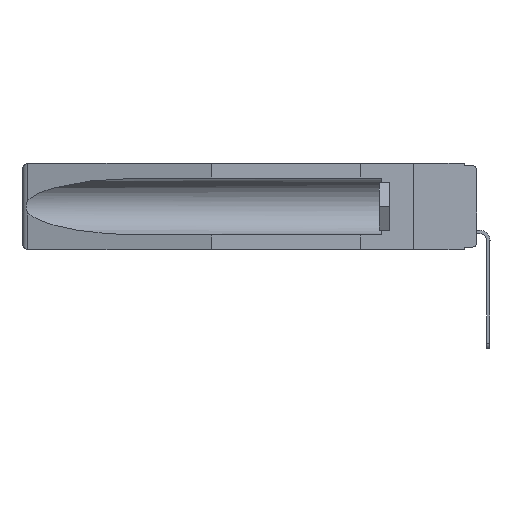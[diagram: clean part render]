
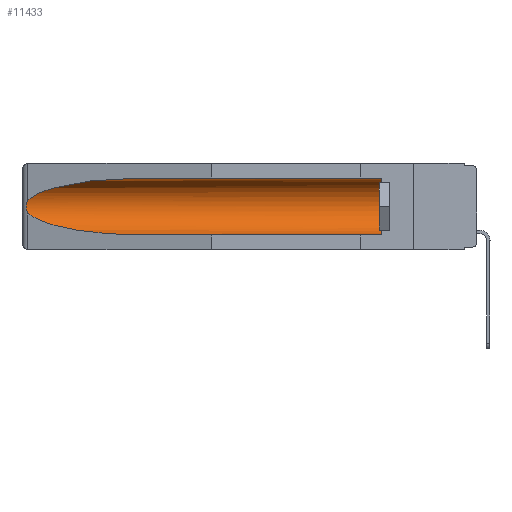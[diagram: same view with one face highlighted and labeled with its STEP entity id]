
A CAD part, left-side view. The second image highlights one B-rep face of the part: STEP entity #11433.
In plain terms, the highlighted cylindrical face has radius 2.857 mm (diameter 5.715 mm), a partial arc.
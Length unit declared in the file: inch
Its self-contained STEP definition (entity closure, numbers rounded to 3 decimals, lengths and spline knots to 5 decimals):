
#317 = VERTEX_POINT ( 'NONE', #20309 ) ;
#428 = DIRECTION ( 'NONE',  ( 0., 0., 1. ) ) ;
#1677 = EDGE_CURVE ( 'NONE', #22620, #21631, #2015, .T. ) ;
#2015 = CIRCLE ( 'NONE', #8006, 0.1125 ) ;
#2112 =( BOUNDED_CURVE ( )  B_SPLINE_CURVE ( 3, ( #15798, #5482, #14286, #9005 ),
 .UNSPECIFIED., .F., .F. ) 
 B_SPLINE_CURVE_WITH_KNOTS ( ( 4, 4 ),
 ( 0.1948, 1.5708 ),
 .UNSPECIFIED. ) 
 CURVE ( )  GEOMETRIC_REPRESENTATION_ITEM ( )  RATIONAL_B_SPLINE_CURVE ( ( 1., 0.848, 0.848, 1. ) ) 
 REPRESENTATION_ITEM ( '' )  );
#2144 = FACE_OUTER_BOUND ( 'NONE', #17711, .T. ) ;
#2998 = CARTESIAN_POINT ( 'NONE',  ( 0.26597, 1.52961, -0.15275 ) ) ;
#3496 = EDGE_CURVE ( 'NONE', #22620, #20487, #17957, .T. ) ;
#4084 = ORIENTED_EDGE ( 'NONE', *, *, #16522, .T. ) ;
#5357 = ORIENTED_EDGE ( 'NONE', *, *, #14694, .T. ) ;
#5415 = DIRECTION ( 'NONE',  ( 0., 0., 1. ) ) ;
#5482 = CARTESIAN_POINT ( 'NONE',  ( 0.25451, 1.48313, -0.24835 ) ) ;
#5709 = B_SPLINE_CURVE_WITH_KNOTS ( 'NONE', 3,
 ( #8035, #2998, #10139, #9798, #9680, #20532, #17052, #16818, #8261, #15075 ),
 .UNSPECIFIED., .F., .F.,
 ( 4, 2, 2, 2, 4 ),
 ( 0., 0.00029, 0.00058, 0.00087, 0.00117 ),
 .UNSPECIFIED. ) ;
#5880 = CARTESIAN_POINT ( 'NONE',  ( 0.155, -0.30754, -0.1715 ) ) ;
#6597 = CARTESIAN_POINT ( 'NONE',  ( 0.25451, 1.48313, -0.09465 ) ) ;
#7158 = VECTOR ( 'NONE', #21571, 39.37008 ) ;
#7311 = ORIENTED_EDGE ( 'NONE', *, *, #19793, .T. ) ;
#7649 =( BOUNDED_CURVE ( )  B_SPLINE_CURVE ( 3, ( #15499, #22643, #6597, #20850 ),
 .UNSPECIFIED., .F., .F. ) 
 B_SPLINE_CURVE_WITH_KNOTS ( ( 4, 4 ),
 ( 4.71239, 6.08839 ),
 .UNSPECIFIED. ) 
 CURVE ( )  GEOMETRIC_REPRESENTATION_ITEM ( )  RATIONAL_B_SPLINE_CURVE ( ( 1., 0.848, 0.848, 1. ) ) 
 REPRESENTATION_ITEM ( '' )  );
#8006 = AXIS2_PLACEMENT_3D ( 'NONE', #18596, #9708, #428 ) ;
#8035 = CARTESIAN_POINT ( 'NONE',  ( 0.26537, 1.52718, -0.14972 ) ) ;
#8261 = CARTESIAN_POINT ( 'NONE',  ( 0.26597, 1.5296, -0.19026 ) ) ;
#8714 = ORIENTED_EDGE ( 'NONE', *, *, #1677, .T. ) ;
#8723 = AXIS2_PLACEMENT_3D ( 'NONE', #5880, #16543, #5415 ) ;
#9005 = CARTESIAN_POINT ( 'NONE',  ( 0.155, 1.07973, -0.284 ) ) ;
#9668 = CARTESIAN_POINT ( 'NONE',  ( 0.155, 0.126, -0.284 ) ) ;
#9680 = CARTESIAN_POINT ( 'NONE',  ( 0.2675, 1.53308, -0.16763 ) ) ;
#9708 = DIRECTION ( 'NONE',  ( 0., -1., 0. ) ) ;
#9798 = CARTESIAN_POINT ( 'NONE',  ( 0.2673, 1.5327, -0.16383 ) ) ;
#10117 = ORIENTED_EDGE ( 'NONE', *, *, #17691, .T. ) ;
#10139 = CARTESIAN_POINT ( 'NONE',  ( 0.26654, 1.53092, -0.15636 ) ) ;
#10431 = VERTEX_POINT ( 'NONE', #20137 ) ;
#10600 = VERTEX_POINT ( 'NONE', #17464 ) ;
#11433 = ADVANCED_FACE ( 'NONE', ( #2144 ), #18174, .F. ) ;
#12569 = CARTESIAN_POINT ( 'NONE',  ( 0.155, -0.30754, -0.284 ) ) ;
#14286 = CARTESIAN_POINT ( 'NONE',  ( 0.21114, 1.30732, -0.284 ) ) ;
#14694 = EDGE_CURVE ( 'NONE', #10600, #10431, #5709, .T. ) ;
#15075 = CARTESIAN_POINT ( 'NONE',  ( 0.26537, 1.52718, -0.19328 ) ) ;
#15499 = CARTESIAN_POINT ( 'NONE',  ( 0.155, 1.07973, -0.059 ) ) ;
#15543 = CARTESIAN_POINT ( 'NONE',  ( 0.155, -0.30754, -0.059 ) ) ;
#15798 = CARTESIAN_POINT ( 'NONE',  ( 0.26537, 1.52718, -0.19328 ) ) ;
#16522 = EDGE_CURVE ( 'NONE', #317, #10600, #7649, .T. ) ;
#16543 = DIRECTION ( 'NONE',  ( 0., 1., 0. ) ) ;
#16818 = CARTESIAN_POINT ( 'NONE',  ( 0.26655, 1.53094, -0.18657 ) ) ;
#17052 = CARTESIAN_POINT ( 'NONE',  ( 0.2673, 1.53269, -0.17917 ) ) ;
#17302 = DIRECTION ( 'NONE',  ( 0., 1., 0. ) ) ;
#17464 = CARTESIAN_POINT ( 'NONE',  ( 0.26537, 1.52718, -0.14972 ) ) ;
#17691 = EDGE_CURVE ( 'NONE', #21631, #317, #19683, .T. ) ;
#17711 = EDGE_LOOP ( 'NONE', ( #4084, #5357, #7311, #18064, #8714, #10117 ) ) ;
#17851 = VECTOR ( 'NONE', #17302, 39.37008 ) ;
#17957 = LINE ( 'NONE', #12569, #7158 ) ;
#18064 = ORIENTED_EDGE ( 'NONE', *, *, #3496, .F. ) ;
#18174 = CYLINDRICAL_SURFACE ( 'NONE', #8723, 0.1125 ) ;
#18596 = CARTESIAN_POINT ( 'NONE',  ( 0.155, 0.126, -0.1715 ) ) ;
#19683 = LINE ( 'NONE', #15543, #17851 ) ;
#19793 = EDGE_CURVE ( 'NONE', #10431, #20487, #2112, .T. ) ;
#19962 = CARTESIAN_POINT ( 'NONE',  ( 0.155, 1.07973, -0.284 ) ) ;
#20137 = CARTESIAN_POINT ( 'NONE',  ( 0.26537, 1.52718, -0.19328 ) ) ;
#20309 = CARTESIAN_POINT ( 'NONE',  ( 0.155, 1.07973, -0.059 ) ) ;
#20487 = VERTEX_POINT ( 'NONE', #19962 ) ;
#20532 = CARTESIAN_POINT ( 'NONE',  ( 0.2675, 1.53308, -0.17534 ) ) ;
#20850 = CARTESIAN_POINT ( 'NONE',  ( 0.26537, 1.52718, -0.14972 ) ) ;
#21553 = CARTESIAN_POINT ( 'NONE',  ( 0.155, 0.126, -0.059 ) ) ;
#21571 = DIRECTION ( 'NONE',  ( 0., 1., 0. ) ) ;
#21631 = VERTEX_POINT ( 'NONE', #21553 ) ;
#22620 = VERTEX_POINT ( 'NONE', #9668 ) ;
#22643 = CARTESIAN_POINT ( 'NONE',  ( 0.21114, 1.30732, -0.059 ) ) ;
